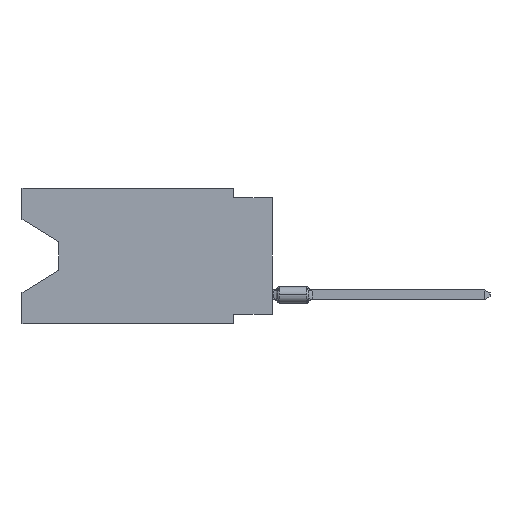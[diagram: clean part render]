
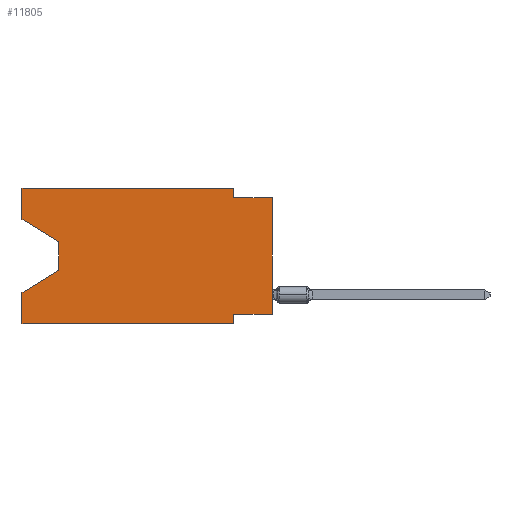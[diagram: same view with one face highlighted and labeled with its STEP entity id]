
A CAD part, left-side view. The second image highlights one B-rep face of the part: STEP entity #11805.
In plain terms, the highlighted planar face has unit normal (-1, 0, 0).
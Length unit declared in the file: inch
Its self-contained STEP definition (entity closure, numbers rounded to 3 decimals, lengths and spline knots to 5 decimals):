
#57 = DIRECTION ( 'NONE',  ( 0., -1., 0. ) ) ;
#94 = VECTOR ( 'NONE', #24386, 39.37008 ) ;
#108 = VERTEX_POINT ( 'NONE', #2231 ) ;
#195 = LINE ( 'NONE', #17116, #11101 ) ;
#233 = VECTOR ( 'NONE', #15240, 39.37008 ) ;
#369 = EDGE_CURVE ( 'NONE', #12041, #19007, #24526, .T. ) ;
#682 = DIRECTION ( 'NONE',  ( 0., -0.855, -0.519 ) ) ;
#1181 = ORIENTED_EDGE ( 'NONE', *, *, #12678, .F. ) ;
#1260 = VERTEX_POINT ( 'NONE', #8669 ) ;
#1267 = ORIENTED_EDGE ( 'NONE', *, *, #21016, .T. ) ;
#1581 = CARTESIAN_POINT ( 'NONE',  ( 0., 0.55, -0.212 ) ) ;
#1688 = EDGE_CURVE ( 'NONE', #20806, #1260, #19037, .T. ) ;
#2231 = CARTESIAN_POINT ( 'NONE',  ( 0., 0.55, -0.212 ) ) ;
#2446 = ORIENTED_EDGE ( 'NONE', *, *, #22720, .F. ) ;
#2515 = LINE ( 'NONE', #6794, #233 ) ;
#2637 = CARTESIAN_POINT ( 'NONE',  ( 0., 0.645, -0.08025 ) ) ;
#2724 = VERTEX_POINT ( 'NONE', #25770 ) ;
#2917 = DIRECTION ( 'NONE',  ( 0., -1., 0. ) ) ;
#3469 = LINE ( 'NONE', #11908, #12197 ) ;
#3962 = ORIENTED_EDGE ( 'NONE', *, *, #9749, .F. ) ;
#4264 = ORIENTED_EDGE ( 'NONE', *, *, #22329, .T. ) ;
#4374 = CARTESIAN_POINT ( 'NONE',  ( 0., 0., -0.025 ) ) ;
#4541 = PLANE ( 'NONE',  #14283 ) ;
#4619 = DIRECTION ( 'NONE',  ( 0., 0., 1. ) ) ;
#4681 = ORIENTED_EDGE ( 'NONE', *, *, #9188, .T. ) ;
#4690 = CARTESIAN_POINT ( 'NONE',  ( 0., 0.1, -0.325 ) ) ;
#4995 = CARTESIAN_POINT ( 'NONE',  ( 0., 0.1, -0.35 ) ) ;
#5395 = CARTESIAN_POINT ( 'NONE',  ( 0., 0., -0.325 ) ) ;
#5710 = VERTEX_POINT ( 'NONE', #22603 ) ;
#5782 = ORIENTED_EDGE ( 'NONE', *, *, #369, .F. ) ;
#6304 = VECTOR ( 'NONE', #21427, 39.37008 ) ;
#6670 = EDGE_CURVE ( 'NONE', #1260, #8649, #195, .T. ) ;
#6794 = CARTESIAN_POINT ( 'NONE',  ( 0., 0.1, 0. ) ) ;
#6958 = VECTOR ( 'NONE', #2917, 39.37008 ) ;
#7380 = VERTEX_POINT ( 'NONE', #13573 ) ;
#7521 = CARTESIAN_POINT ( 'NONE',  ( 0., 0.1, -0.35 ) ) ;
#8649 = VERTEX_POINT ( 'NONE', #26754 ) ;
#8669 = CARTESIAN_POINT ( 'NONE',  ( 0., 0.645, 0. ) ) ;
#9188 = EDGE_CURVE ( 'NONE', #108, #2724, #10277, .T. ) ;
#9532 = DIRECTION ( 'NONE',  ( 0., 0., 1. ) ) ;
#9641 = CARTESIAN_POINT ( 'NONE',  ( 0., 0., -0.325 ) ) ;
#9749 = EDGE_CURVE ( 'NONE', #8649, #5710, #2515, .T. ) ;
#10277 = LINE ( 'NONE', #1581, #11599 ) ;
#10611 = CARTESIAN_POINT ( 'NONE',  ( 0., 0.645, 0. ) ) ;
#11101 = VECTOR ( 'NONE', #57, 39.37008 ) ;
#11266 = VERTEX_POINT ( 'NONE', #7521 ) ;
#11484 = CARTESIAN_POINT ( 'NONE',  ( 0., 0.645, -0.35 ) ) ;
#11599 = VECTOR ( 'NONE', #19025, 39.37008 ) ;
#11805 = ADVANCED_FACE ( 'NONE', ( #21179 ), #4541, .F. ) ;
#11908 = CARTESIAN_POINT ( 'NONE',  ( 0., 0.55, -0.138 ) ) ;
#11953 = ORIENTED_EDGE ( 'NONE', *, *, #13272, .T. ) ;
#12041 = VERTEX_POINT ( 'NONE', #9641 ) ;
#12197 = VECTOR ( 'NONE', #22588, 39.37008 ) ;
#12678 = EDGE_CURVE ( 'NONE', #5710, #7380, #25591, .T. ) ;
#13087 = VECTOR ( 'NONE', #4619, 39.37008 ) ;
#13232 = ORIENTED_EDGE ( 'NONE', *, *, #1688, .F. ) ;
#13272 = EDGE_CURVE ( 'NONE', #17008, #108, #3469, .T. ) ;
#13441 = DIRECTION ( 'NONE',  ( 0., 0., -1. ) ) ;
#13573 = CARTESIAN_POINT ( 'NONE',  ( 0., 0., -0.025 ) ) ;
#14283 = AXIS2_PLACEMENT_3D ( 'NONE', #10611, #19093, #16367 ) ;
#14284 = CARTESIAN_POINT ( 'NONE',  ( 0., 0.645, -0.08025 ) ) ;
#14687 = ORIENTED_EDGE ( 'NONE', *, *, #6670, .F. ) ;
#15240 = DIRECTION ( 'NONE',  ( 0., 0., -1. ) ) ;
#16367 = DIRECTION ( 'NONE',  ( 0., 0., -1. ) ) ;
#16692 = CARTESIAN_POINT ( 'NONE',  ( 0., 0.645, 0. ) ) ;
#17008 = VERTEX_POINT ( 'NONE', #25553 ) ;
#17116 = CARTESIAN_POINT ( 'NONE',  ( 0., 0.645, 0. ) ) ;
#17884 = LINE ( 'NONE', #4995, #21952 ) ;
#18592 = ORIENTED_EDGE ( 'NONE', *, *, #24176, .F. ) ;
#19007 = VERTEX_POINT ( 'NONE', #4690 ) ;
#19025 = DIRECTION ( 'NONE',  ( 0., 0.855, -0.519 ) ) ;
#19037 = LINE ( 'NONE', #16692, #13087 ) ;
#19093 = DIRECTION ( 'NONE',  ( 1., 0., 0. ) ) ;
#19315 = VECTOR ( 'NONE', #9532, 39.37008 ) ;
#19386 = CARTESIAN_POINT ( 'NONE',  ( 0., 0.645, 0. ) ) ;
#19622 = ORIENTED_EDGE ( 'NONE', *, *, #21145, .T. ) ;
#19744 = VECTOR ( 'NONE', #21728, 39.37008 ) ;
#20806 = VERTEX_POINT ( 'NONE', #14284 ) ;
#21016 = EDGE_CURVE ( 'NONE', #20806, #17008, #23836, .T. ) ;
#21145 = EDGE_CURVE ( 'NONE', #12041, #7380, #24660, .T. ) ;
#21179 = FACE_OUTER_BOUND ( 'NONE', #26215, .T. ) ;
#21427 = DIRECTION ( 'NONE',  ( 0., -1., 0. ) ) ;
#21632 = LINE ( 'NONE', #11484, #6958 ) ;
#21661 = VERTEX_POINT ( 'NONE', #22418 ) ;
#21728 = DIRECTION ( 'NONE',  ( 0., 0., 1. ) ) ;
#21952 = VECTOR ( 'NONE', #13441, 39.37008 ) ;
#22329 = EDGE_CURVE ( 'NONE', #21661, #11266, #21632, .T. ) ;
#22418 = CARTESIAN_POINT ( 'NONE',  ( 0., 0.645, -0.35 ) ) ;
#22588 = DIRECTION ( 'NONE',  ( 0., 0., -1. ) ) ;
#22603 = CARTESIAN_POINT ( 'NONE',  ( 0., 0.1, -0.025 ) ) ;
#22720 = EDGE_CURVE ( 'NONE', #21661, #2724, #26025, .T. ) ;
#23836 = LINE ( 'NONE', #2637, #25507 ) ;
#24176 = EDGE_CURVE ( 'NONE', #19007, #11266, #17884, .T. ) ;
#24249 = CARTESIAN_POINT ( 'NONE',  ( 0., 0., 0. ) ) ;
#24386 = DIRECTION ( 'NONE',  ( 0., 1., 0. ) ) ;
#24526 = LINE ( 'NONE', #5395, #94 ) ;
#24660 = LINE ( 'NONE', #24249, #19315 ) ;
#25507 = VECTOR ( 'NONE', #682, 39.37008 ) ;
#25553 = CARTESIAN_POINT ( 'NONE',  ( 0., 0.55, -0.138 ) ) ;
#25591 = LINE ( 'NONE', #4374, #6304 ) ;
#25770 = CARTESIAN_POINT ( 'NONE',  ( 0., 0.645, -0.26975 ) ) ;
#26025 = LINE ( 'NONE', #19386, #19744 ) ;
#26215 = EDGE_LOOP ( 'NONE', ( #1267, #11953, #4681, #2446, #4264, #18592, #5782, #19622, #1181, #3962, #14687, #13232 ) ) ;
#26754 = CARTESIAN_POINT ( 'NONE',  ( 0., 0.1, 0. ) ) ;
